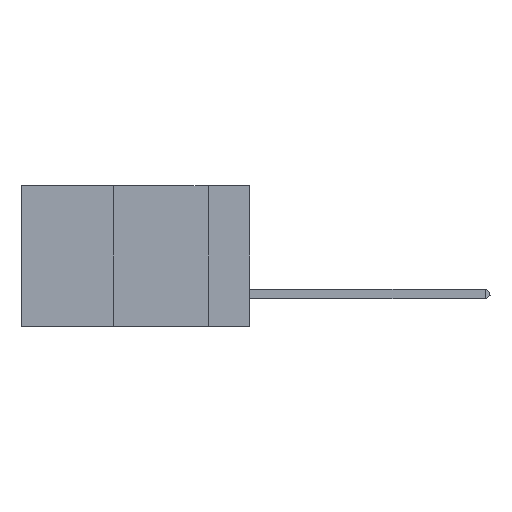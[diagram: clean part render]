
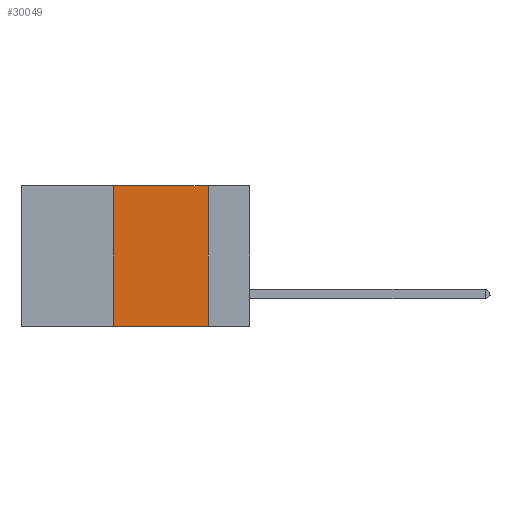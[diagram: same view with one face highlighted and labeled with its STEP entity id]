
A CAD part, left-side view. The second image highlights one B-rep face of the part: STEP entity #30049.
In plain terms, the highlighted planar face has unit normal (-1, 0, 0).
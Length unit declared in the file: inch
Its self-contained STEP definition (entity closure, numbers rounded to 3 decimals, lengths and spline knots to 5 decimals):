
#1856 = EDGE_LOOP ( 'NONE', ( #28282, #42217, #42196, #22300 ) ) ;
#2587 = PLANE ( 'NONE',  #38514 ) ;
#5525 = CARTESIAN_POINT ( 'NONE',  ( 0., 0.6, 0. ) ) ;
#5965 = DIRECTION ( 'NONE',  ( 1., 0., 0. ) ) ;
#5995 = DIRECTION ( 'NONE',  ( 0., 0., 1. ) ) ;
#6561 = VECTOR ( 'NONE', #15820, 39.37008 ) ;
#11158 = CARTESIAN_POINT ( 'NONE',  ( 0., 0.11, 0. ) ) ;
#11331 = VERTEX_POINT ( 'NONE', #41797 ) ;
#12963 = CARTESIAN_POINT ( 'NONE',  ( 0., 0.6, 0. ) ) ;
#14624 = CARTESIAN_POINT ( 'NONE',  ( 0., 0.11, -0.37 ) ) ;
#14792 = FACE_OUTER_BOUND ( 'NONE', #1856, .T. ) ;
#15485 = LINE ( 'NONE', #11158, #19769 ) ;
#15820 = DIRECTION ( 'NONE',  ( 0., -1., 0. ) ) ;
#16243 = VERTEX_POINT ( 'NONE', #14624 ) ;
#19576 = CARTESIAN_POINT ( 'NONE',  ( 0., 0.36, 0. ) ) ;
#19769 = VECTOR ( 'NONE', #34431, 39.37008 ) ;
#21591 = EDGE_CURVE ( 'NONE', #11331, #38952, #41275, .T. ) ;
#21632 = DIRECTION ( 'NONE',  ( 0., -1., 0. ) ) ;
#22300 = ORIENTED_EDGE ( 'NONE', *, *, #24508, .T. ) ;
#24508 = EDGE_CURVE ( 'NONE', #38285, #16243, #31320, .T. ) ;
#25999 = VECTOR ( 'NONE', #21632, 39.37008 ) ;
#28282 = ORIENTED_EDGE ( 'NONE', *, *, #40816, .F. ) ;
#28982 = EDGE_CURVE ( 'NONE', #38285, #11331, #30873, .T. ) ;
#30049 = ADVANCED_FACE ( 'NONE', ( #14792 ), #2587, .F. ) ;
#30873 = LINE ( 'NONE', #19576, #36194 ) ;
#31268 = CARTESIAN_POINT ( 'NONE',  ( 0., 0.6, -0.37 ) ) ;
#31320 = LINE ( 'NONE', #31268, #25999 ) ;
#34431 = DIRECTION ( 'NONE',  ( 0., 0., -1. ) ) ;
#36194 = VECTOR ( 'NONE', #5995, 39.37008 ) ;
#37084 = DIRECTION ( 'NONE',  ( 0., 0., -1. ) ) ;
#38285 = VERTEX_POINT ( 'NONE', #41372 ) ;
#38488 = CARTESIAN_POINT ( 'NONE',  ( 0., 0.11, 0. ) ) ;
#38514 = AXIS2_PLACEMENT_3D ( 'NONE', #12963, #5965, #37084 ) ;
#38952 = VERTEX_POINT ( 'NONE', #38488 ) ;
#40816 = EDGE_CURVE ( 'NONE', #38952, #16243, #15485, .T. ) ;
#41275 = LINE ( 'NONE', #5525, #6561 ) ;
#41372 = CARTESIAN_POINT ( 'NONE',  ( 0., 0.36, -0.37 ) ) ;
#41797 = CARTESIAN_POINT ( 'NONE',  ( 0., 0.36, 0. ) ) ;
#42196 = ORIENTED_EDGE ( 'NONE', *, *, #28982, .F. ) ;
#42217 = ORIENTED_EDGE ( 'NONE', *, *, #21591, .F. ) ;
